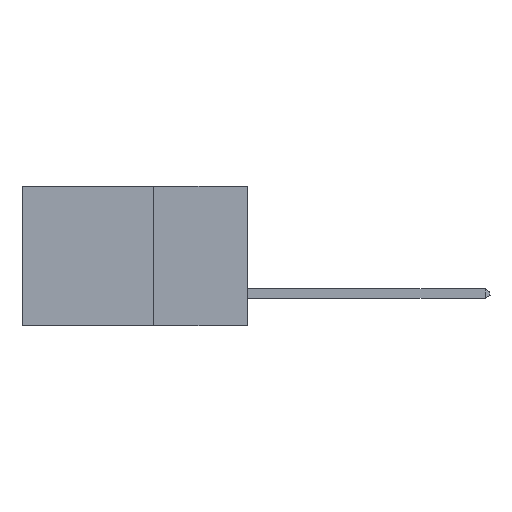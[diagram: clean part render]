
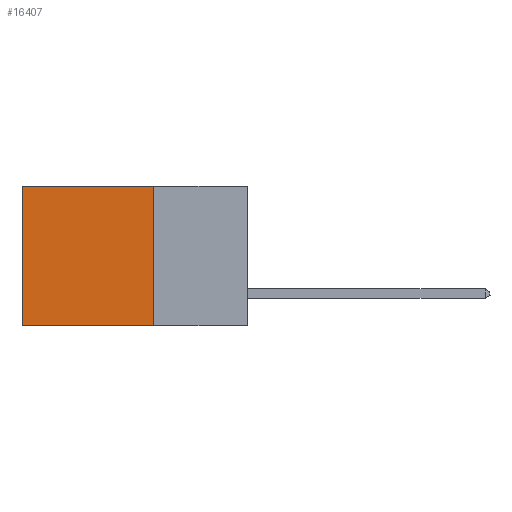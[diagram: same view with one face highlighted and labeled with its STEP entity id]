
A CAD part, left-side view. The second image highlights one B-rep face of the part: STEP entity #16407.
In plain terms, the highlighted planar face has unit normal (-1, 0, 0).
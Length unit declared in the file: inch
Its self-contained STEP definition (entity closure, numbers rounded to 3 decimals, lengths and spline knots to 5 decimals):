
#173 = CARTESIAN_POINT ( 'NONE',  ( 0.298, 0.25, 0. ) ) ;
#1824 = FACE_OUTER_BOUND ( 'NONE', #10554, .T. ) ;
#2412 = VERTEX_POINT ( 'NONE', #18157 ) ;
#2517 = CARTESIAN_POINT ( 'NONE',  ( 0.298, 0.25, 0. ) ) ;
#3701 = DIRECTION ( 'NONE',  ( 0., 1., 0. ) ) ;
#3908 = VECTOR ( 'NONE', #4111, 39.37008 ) ;
#4111 = DIRECTION ( 'NONE',  ( 0., 1., 0. ) ) ;
#4350 = CARTESIAN_POINT ( 'NONE',  ( 0.298, 0.25, 0. ) ) ;
#4371 = DIRECTION ( 'NONE',  ( 1., 0., 0. ) ) ;
#7237 = EDGE_CURVE ( 'NONE', #20243, #18563, #19685, .T. ) ;
#7812 = LINE ( 'NONE', #24747, #3908 ) ;
#8804 = AXIS2_PLACEMENT_3D ( 'NONE', #173, #4371, #12918 ) ;
#10220 = PLANE ( 'NONE',  #8804 ) ;
#10520 = DIRECTION ( 'NONE',  ( 0., 0., -1. ) ) ;
#10554 = EDGE_LOOP ( 'NONE', ( #16727, #20735, #25556, #15718 ) ) ;
#10601 = VECTOR ( 'NONE', #10520, 39.37008 ) ;
#12918 = DIRECTION ( 'NONE',  ( 0., 0., -1. ) ) ;
#14013 = LINE ( 'NONE', #20418, #21500 ) ;
#14019 = CARTESIAN_POINT ( 'NONE',  ( 0.298, 0.25, -0.37 ) ) ;
#14060 = CARTESIAN_POINT ( 'NONE',  ( 0.298, 0.25, -0.37 ) ) ;
#15718 = ORIENTED_EDGE ( 'NONE', *, *, #23669, .T. ) ;
#16407 = ADVANCED_FACE ( 'NONE', ( #1824 ), #10220, .F. ) ;
#16727 = ORIENTED_EDGE ( 'NONE', *, *, #17831, .T. ) ;
#17831 = EDGE_CURVE ( 'NONE', #2412, #25584, #14013, .T. ) ;
#18157 = CARTESIAN_POINT ( 'NONE',  ( 0.298, 0.6, 0. ) ) ;
#18285 = CARTESIAN_POINT ( 'NONE',  ( 0.298, 0.6, -0.37 ) ) ;
#18563 = VERTEX_POINT ( 'NONE', #14019 ) ;
#19685 = LINE ( 'NONE', #2517, #10601 ) ;
#20243 = VERTEX_POINT ( 'NONE', #4350 ) ;
#20418 = CARTESIAN_POINT ( 'NONE',  ( 0.298, 0.6, 0. ) ) ;
#20735 = ORIENTED_EDGE ( 'NONE', *, *, #24979, .F. ) ;
#21500 = VECTOR ( 'NONE', #26492, 39.37008 ) ;
#23669 = EDGE_CURVE ( 'NONE', #20243, #2412, #7812, .T. ) ;
#23965 = LINE ( 'NONE', #14060, #25252 ) ;
#24747 = CARTESIAN_POINT ( 'NONE',  ( 0.298, 0.25, 0. ) ) ;
#24979 = EDGE_CURVE ( 'NONE', #18563, #25584, #23965, .T. ) ;
#25252 = VECTOR ( 'NONE', #3701, 39.37008 ) ;
#25556 = ORIENTED_EDGE ( 'NONE', *, *, #7237, .F. ) ;
#25584 = VERTEX_POINT ( 'NONE', #18285 ) ;
#26492 = DIRECTION ( 'NONE',  ( 0., 0., -1. ) ) ;
